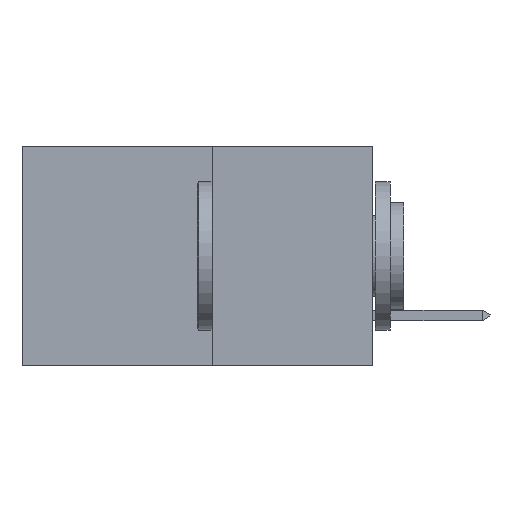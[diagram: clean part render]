
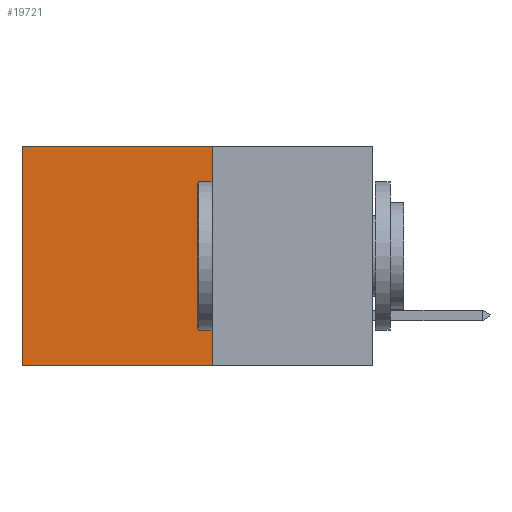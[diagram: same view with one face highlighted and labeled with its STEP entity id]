
A CAD part, left-side view. The second image highlights one B-rep face of the part: STEP entity #19721.
In plain terms, the highlighted planar face has unit normal (-1, 0, 0).
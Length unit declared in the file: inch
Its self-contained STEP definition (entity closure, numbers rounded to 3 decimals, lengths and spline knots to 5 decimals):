
#605 = DIRECTION ( 'NONE',  ( 1., 0., 0. ) ) ;
#825 = VECTOR ( 'NONE', #5347, 39.37008 ) ;
#1341 = LINE ( 'NONE', #15009, #825 ) ;
#2864 = CARTESIAN_POINT ( 'NONE',  ( 0.277, 0.27, -0.37 ) ) ;
#3747 = VERTEX_POINT ( 'NONE', #10041 ) ;
#3751 = VECTOR ( 'NONE', #13068, 39.37008 ) ;
#3757 = PLANE ( 'NONE',  #6900 ) ;
#4679 = LINE ( 'NONE', #11648, #8497 ) ;
#5347 = DIRECTION ( 'NONE',  ( 0., 0., -1. ) ) ;
#5974 = ORIENTED_EDGE ( 'NONE', *, *, #16814, .F. ) ;
#6900 = AXIS2_PLACEMENT_3D ( 'NONE', #10319, #605, #11964 ) ;
#7305 = EDGE_CURVE ( 'NONE', #10995, #8111, #4679, .T. ) ;
#8111 = VERTEX_POINT ( 'NONE', #18363 ) ;
#8497 = VECTOR ( 'NONE', #10731, 39.37008 ) ;
#10041 = CARTESIAN_POINT ( 'NONE',  ( 0.277, 0.27, 0. ) ) ;
#10319 = CARTESIAN_POINT ( 'NONE',  ( 0.277, 0.27, -0.37 ) ) ;
#10731 = DIRECTION ( 'NONE',  ( 0., 1., 0. ) ) ;
#10960 = VERTEX_POINT ( 'NONE', #18908 ) ;
#10995 = VERTEX_POINT ( 'NONE', #2864 ) ;
#11648 = CARTESIAN_POINT ( 'NONE',  ( 0.277, 0.27, -0.37 ) ) ;
#11849 = LINE ( 'NONE', #16321, #3751 ) ;
#11964 = DIRECTION ( 'NONE',  ( 0., 0., -1. ) ) ;
#12133 = EDGE_CURVE ( 'NONE', #10960, #8111, #16878, .T. ) ;
#13068 = DIRECTION ( 'NONE',  ( 0., 1., 0. ) ) ;
#13165 = ORIENTED_EDGE ( 'NONE', *, *, #12133, .T. ) ;
#13389 = DIRECTION ( 'NONE',  ( 0., 0., -1. ) ) ;
#14118 = EDGE_CURVE ( 'NONE', #3747, #10960, #11849, .T. ) ;
#14851 = CARTESIAN_POINT ( 'NONE',  ( 0.277, 0.59, -0.37 ) ) ;
#15009 = CARTESIAN_POINT ( 'NONE',  ( 0.277, 0.27, -0.37 ) ) ;
#15558 = FACE_OUTER_BOUND ( 'NONE', #19444, .T. ) ;
#16039 = ORIENTED_EDGE ( 'NONE', *, *, #14118, .T. ) ;
#16321 = CARTESIAN_POINT ( 'NONE',  ( 0.277, 0.27, 0. ) ) ;
#16814 = EDGE_CURVE ( 'NONE', #3747, #10995, #1341, .T. ) ;
#16878 = LINE ( 'NONE', #14851, #20719 ) ;
#17336 = ORIENTED_EDGE ( 'NONE', *, *, #7305, .F. ) ;
#18363 = CARTESIAN_POINT ( 'NONE',  ( 0.277, 0.59, -0.37 ) ) ;
#18908 = CARTESIAN_POINT ( 'NONE',  ( 0.277, 0.59, 0. ) ) ;
#19444 = EDGE_LOOP ( 'NONE', ( #13165, #17336, #5974, #16039 ) ) ;
#19721 = ADVANCED_FACE ( 'NONE', ( #15558 ), #3757, .F. ) ;
#20719 = VECTOR ( 'NONE', #13389, 39.37008 ) ;
